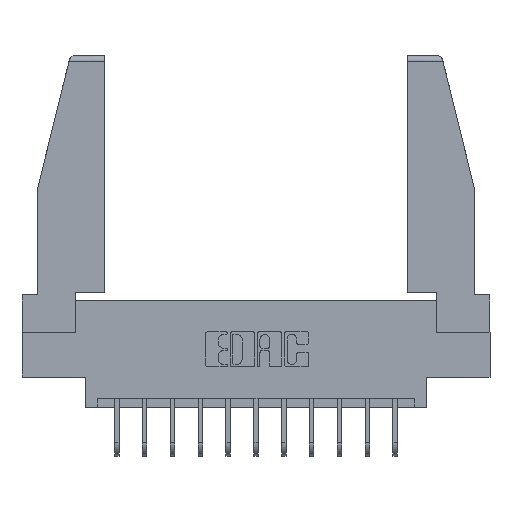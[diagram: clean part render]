
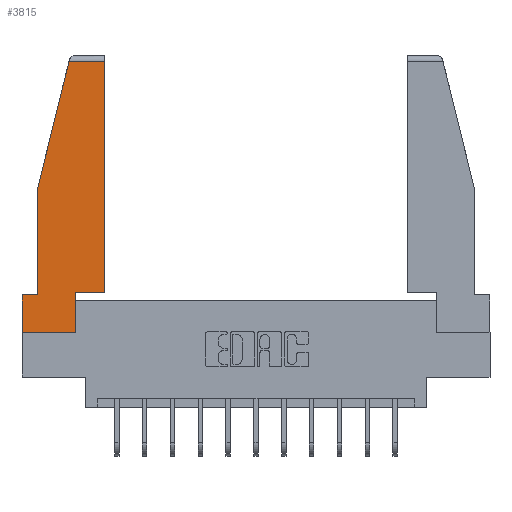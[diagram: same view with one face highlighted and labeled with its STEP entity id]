
A CAD part, top view. The second image highlights one B-rep face of the part: STEP entity #3815.
In plain terms, the highlighted planar face has unit normal (0, 0, 1).
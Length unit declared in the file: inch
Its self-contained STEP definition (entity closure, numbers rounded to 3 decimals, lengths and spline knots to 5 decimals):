
#28 = VECTOR ( 'NONE', #13152, 39.37008 ) ;
#500 = VERTEX_POINT ( 'NONE', #8776 ) ;
#661 = CARTESIAN_POINT ( 'NONE',  ( 0.086, 0.8, 0. ) ) ;
#738 = VECTOR ( 'NONE', #13808, 39.37008 ) ;
#991 = CARTESIAN_POINT ( 'NONE',  ( 0.461, 0.223, 0. ) ) ;
#1506 = EDGE_CURVE ( 'NONE', #500, #12550, #5023, .T. ) ;
#1600 = CARTESIAN_POINT ( 'NONE',  ( 0.271, 1.55, 0. ) ) ;
#1660 = EDGE_CURVE ( 'NONE', #13151, #12981, #13296, .T. ) ;
#2008 = DIRECTION ( 'NONE',  ( 0., 1., 0. ) ) ;
#2118 = AXIS2_PLACEMENT_3D ( 'NONE', #6827, #6975, #3666 ) ;
#2490 = ORIENTED_EDGE ( 'NONE', *, *, #10277, .T. ) ;
#2527 = LINE ( 'NONE', #13181, #14386 ) ;
#2562 = CARTESIAN_POINT ( 'NONE',  ( 0., 0.21, 0. ) ) ;
#3666 = DIRECTION ( 'NONE',  ( 1., 0., 0. ) ) ;
#3782 = LINE ( 'NONE', #12631, #738 ) ;
#3805 = ORIENTED_EDGE ( 'NONE', *, *, #14109, .T. ) ;
#3815 = ADVANCED_FACE ( 'NONE', ( #7750 ), #14621, .T. ) ;
#3854 = LINE ( 'NONE', #12569, #12282 ) ;
#4004 = VERTEX_POINT ( 'NONE', #10997 ) ;
#4036 = EDGE_CURVE ( 'NONE', #4004, #7689, #12406, .T. ) ;
#4143 = ORIENTED_EDGE ( 'NONE', *, *, #1660, .T. ) ;
#4170 = ORIENTED_EDGE ( 'NONE', *, *, #4036, .T. ) ;
#4259 = LINE ( 'NONE', #12965, #6232 ) ;
#4619 = EDGE_CURVE ( 'NONE', #12981, #500, #2527, .T. ) ;
#5023 = LINE ( 'NONE', #1600, #28 ) ;
#5674 = ORIENTED_EDGE ( 'NONE', *, *, #4619, .T. ) ;
#5784 = VERTEX_POINT ( 'NONE', #12897 ) ;
#6232 = VECTOR ( 'NONE', #9546, 39.37008 ) ;
#6359 = EDGE_CURVE ( 'NONE', #11262, #4004, #4259, .T. ) ;
#6827 = CARTESIAN_POINT ( 'NONE',  ( 0., 0., 0. ) ) ;
#6975 = DIRECTION ( 'NONE',  ( 0., 0., 1. ) ) ;
#7497 = VERTEX_POINT ( 'NONE', #7608 ) ;
#7598 = CARTESIAN_POINT ( 'NONE',  ( 0., 0.21, 0. ) ) ;
#7608 = CARTESIAN_POINT ( 'NONE',  ( 0.297, 0.223, 0. ) ) ;
#7689 = VERTEX_POINT ( 'NONE', #10729 ) ;
#7750 = FACE_OUTER_BOUND ( 'NONE', #14453, .T. ) ;
#7794 = EDGE_CURVE ( 'NONE', #7497, #13151, #3854, .T. ) ;
#8013 = VECTOR ( 'NONE', #11458, 39.37008 ) ;
#8635 = VECTOR ( 'NONE', #12459, 39.37008 ) ;
#8739 = LINE ( 'NONE', #13918, #8013 ) ;
#8776 = CARTESIAN_POINT ( 'NONE',  ( 0.2636, 1.52, 0. ) ) ;
#8946 = ORIENTED_EDGE ( 'NONE', *, *, #7794, .T. ) ;
#9546 = DIRECTION ( 'NONE',  ( 0., -1., 0. ) ) ;
#9701 = DIRECTION ( 'NONE',  ( -1., 0., 0. ) ) ;
#10100 = CARTESIAN_POINT ( 'NONE',  ( 0.461, 0.223, 0. ) ) ;
#10206 = CARTESIAN_POINT ( 'NONE',  ( 0., 0., 0. ) ) ;
#10224 = VECTOR ( 'NONE', #2008, 39.37008 ) ;
#10264 = DIRECTION ( 'NONE',  ( 1., 0., 0. ) ) ;
#10277 = EDGE_CURVE ( 'NONE', #7689, #7497, #8739, .T. ) ;
#10661 = CARTESIAN_POINT ( 'NONE',  ( 0.461, 1.52, 0. ) ) ;
#10729 = CARTESIAN_POINT ( 'NONE',  ( 0.297, 0., 0. ) ) ;
#10997 = CARTESIAN_POINT ( 'NONE',  ( 0., 0., 0. ) ) ;
#11262 = VERTEX_POINT ( 'NONE', #7598 ) ;
#11458 = DIRECTION ( 'NONE',  ( 0., 1., 0. ) ) ;
#11865 = LINE ( 'NONE', #2562, #13854 ) ;
#11926 = ORIENTED_EDGE ( 'NONE', *, *, #6359, .T. ) ;
#12029 = EDGE_CURVE ( 'NONE', #12550, #5784, #3782, .T. ) ;
#12282 = VECTOR ( 'NONE', #10264, 39.37008 ) ;
#12406 = LINE ( 'NONE', #10206, #8635 ) ;
#12459 = DIRECTION ( 'NONE',  ( 1., 0., 0. ) ) ;
#12550 = VERTEX_POINT ( 'NONE', #661 ) ;
#12569 = CARTESIAN_POINT ( 'NONE',  ( 0.297, 0.223, 0. ) ) ;
#12631 = CARTESIAN_POINT ( 'NONE',  ( 0.086, 0.8, 0. ) ) ;
#12714 = ORIENTED_EDGE ( 'NONE', *, *, #12029, .T. ) ;
#12897 = CARTESIAN_POINT ( 'NONE',  ( 0.086, 0.21, 0. ) ) ;
#12965 = CARTESIAN_POINT ( 'NONE',  ( 0., 0.21, 0. ) ) ;
#12981 = VERTEX_POINT ( 'NONE', #10661 ) ;
#13151 = VERTEX_POINT ( 'NONE', #10100 ) ;
#13152 = DIRECTION ( 'NONE',  ( -0.239, -0.971, 0. ) ) ;
#13181 = CARTESIAN_POINT ( 'NONE',  ( 0., 1.52, 0. ) ) ;
#13296 = LINE ( 'NONE', #991, #10224 ) ;
#13496 = ORIENTED_EDGE ( 'NONE', *, *, #1506, .T. ) ;
#13808 = DIRECTION ( 'NONE',  ( 0., -1., 0. ) ) ;
#13854 = VECTOR ( 'NONE', #14011, 39.37008 ) ;
#13918 = CARTESIAN_POINT ( 'NONE',  ( 0.297, 0., 0. ) ) ;
#14011 = DIRECTION ( 'NONE',  ( -1., 0., 0. ) ) ;
#14109 = EDGE_CURVE ( 'NONE', #5784, #11262, #11865, .T. ) ;
#14386 = VECTOR ( 'NONE', #9701, 39.37008 ) ;
#14453 = EDGE_LOOP ( 'NONE', ( #4143, #5674, #13496, #12714, #3805, #11926, #4170, #2490, #8946 ) ) ;
#14621 = PLANE ( 'NONE',  #2118 ) ;
